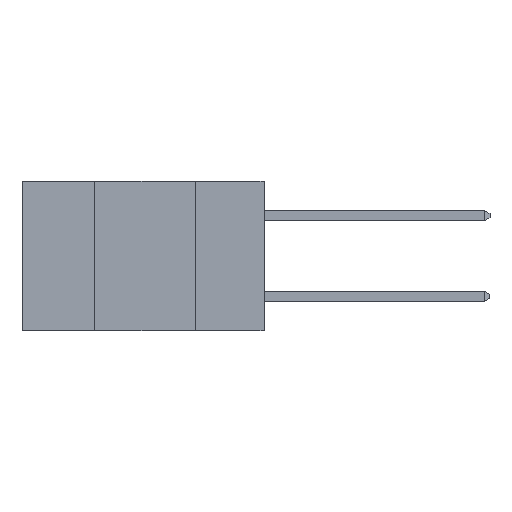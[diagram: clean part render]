
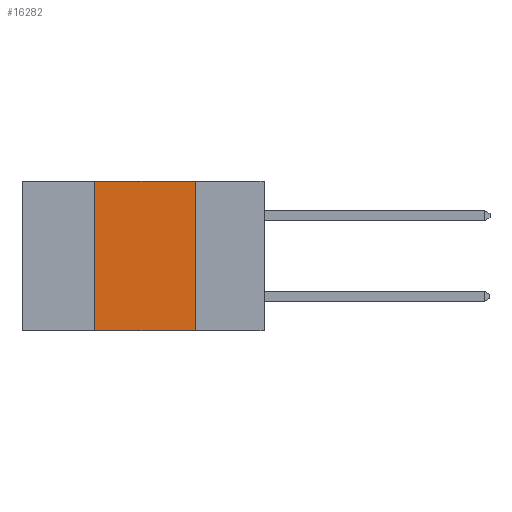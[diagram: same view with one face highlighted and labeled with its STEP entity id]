
A CAD part, left-side view. The second image highlights one B-rep face of the part: STEP entity #16282.
In plain terms, the highlighted planar face has unit normal (-1, 0, 0).
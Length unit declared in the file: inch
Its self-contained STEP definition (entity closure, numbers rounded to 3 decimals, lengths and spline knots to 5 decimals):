
#4 = CARTESIAN_POINT ( 'NONE',  ( 0., 0.6, -0.37 ) ) ;
#1044 = ORIENTED_EDGE ( 'NONE', *, *, #10207, .F. ) ;
#1244 = CARTESIAN_POINT ( 'NONE',  ( 0., 0.6, 0. ) ) ;
#2075 = VECTOR ( 'NONE', #16983, 39.37008 ) ;
#2098 = DIRECTION ( 'NONE',  ( 0., 0., -1. ) ) ;
#2500 = LINE ( 'NONE', #10184, #2075 ) ;
#3076 = EDGE_CURVE ( 'NONE', #17100, #6503, #16684, .T. ) ;
#3198 = ORIENTED_EDGE ( 'NONE', *, *, #3076, .F. ) ;
#3372 = VERTEX_POINT ( 'NONE', #13030 ) ;
#3664 = AXIS2_PLACEMENT_3D ( 'NONE', #1244, #5424, #15209 ) ;
#3673 = EDGE_CURVE ( 'NONE', #11776, #6503, #13814, .T. ) ;
#5424 = DIRECTION ( 'NONE',  ( 1., 0., 0. ) ) ;
#5864 = CARTESIAN_POINT ( 'NONE',  ( 0., 0.6, 0. ) ) ;
#6131 = EDGE_CURVE ( 'NONE', #3372, #17100, #12270, .T. ) ;
#6469 = ORIENTED_EDGE ( 'NONE', *, *, #6131, .F. ) ;
#6503 = VERTEX_POINT ( 'NONE', #14985 ) ;
#7211 = VECTOR ( 'NONE', #8579, 39.37008 ) ;
#7975 = ORIENTED_EDGE ( 'NONE', *, *, #3673, .T. ) ;
#8048 = VECTOR ( 'NONE', #2098, 39.37008 ) ;
#8579 = DIRECTION ( 'NONE',  ( 0., -1., 0. ) ) ;
#9283 = CARTESIAN_POINT ( 'NONE',  ( 0., 0.17, 0. ) ) ;
#10184 = CARTESIAN_POINT ( 'NONE',  ( 0., 0.42, 0. ) ) ;
#10207 = EDGE_CURVE ( 'NONE', #11776, #3372, #2500, .T. ) ;
#11776 = VERTEX_POINT ( 'NONE', #15399 ) ;
#12270 = LINE ( 'NONE', #5864, #7211 ) ;
#13030 = CARTESIAN_POINT ( 'NONE',  ( 0., 0.42, 0. ) ) ;
#13375 = VECTOR ( 'NONE', #15944, 39.37008 ) ;
#13814 = LINE ( 'NONE', #4, #13375 ) ;
#13856 = PLANE ( 'NONE',  #3664 ) ;
#14664 = CARTESIAN_POINT ( 'NONE',  ( 0., 0.17, 0. ) ) ;
#14985 = CARTESIAN_POINT ( 'NONE',  ( 0., 0.17, -0.37 ) ) ;
#15209 = DIRECTION ( 'NONE',  ( 0., 0., -1. ) ) ;
#15399 = CARTESIAN_POINT ( 'NONE',  ( 0., 0.42, -0.37 ) ) ;
#15944 = DIRECTION ( 'NONE',  ( 0., -1., 0. ) ) ;
#16282 = ADVANCED_FACE ( 'NONE', ( #17616 ), #13856, .F. ) ;
#16584 = EDGE_LOOP ( 'NONE', ( #3198, #6469, #1044, #7975 ) ) ;
#16684 = LINE ( 'NONE', #9283, #8048 ) ;
#16983 = DIRECTION ( 'NONE',  ( 0., 0., 1. ) ) ;
#17100 = VERTEX_POINT ( 'NONE', #14664 ) ;
#17616 = FACE_OUTER_BOUND ( 'NONE', #16584, .T. ) ;
